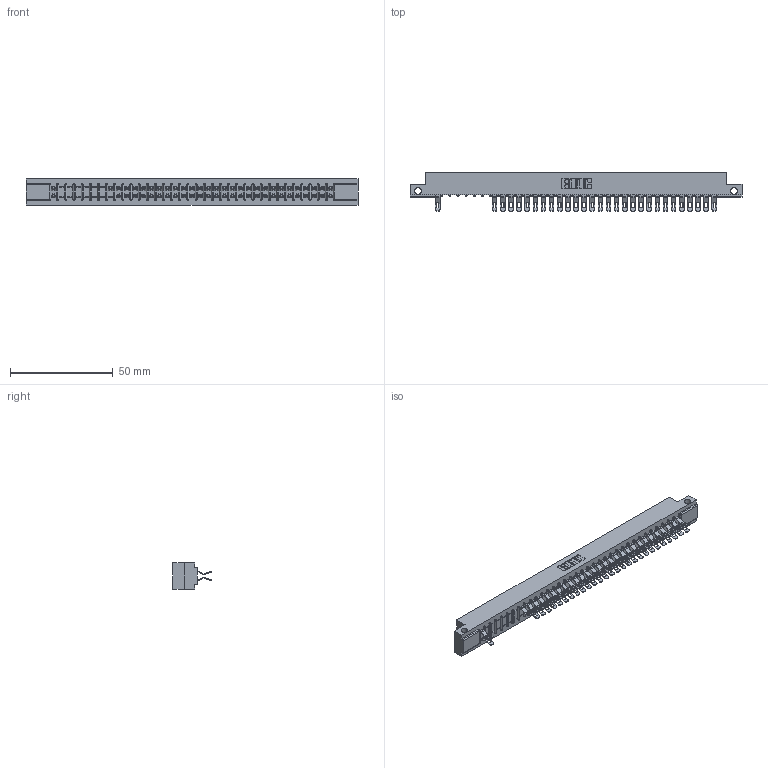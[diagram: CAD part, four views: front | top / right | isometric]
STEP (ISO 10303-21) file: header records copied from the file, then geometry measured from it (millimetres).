
FILE_DESCRIPTION (( 'STEP AP203' ), '1' );
FILE_NAME ('307-070-555-212.STEP', '2018-08-06T13:10:49', ( '' ), ( '' ), 'SwSTEP 2.0', 'SolidWorks 2016', '' );
FILE_SCHEMA (( 'CONFIG_CONTROL_DESIGN' ));
Length unit declared in the file: inch
Products named in the file (3): 307 Part_.128 Dia Side Mounting Holes; 307-290-001_555; 307-070-555-212
Assembly tree (58 placements, depth 2):
  307-070-555-212
    307 Part_.128 Dia Side Mounting Holes
    307-290-001_555  x57
Bounding box: 161.7 x 18.75 x 12.7 mm (x, y, z)
Volume: 17004.3 mm3; surface area: 20487.2 mm2
Topology: 58 solids, 58 shells, 3761 faces, 11056 edges, 7196 vertices
Faces by surface type: plane 2086, cylinder 1603, sphere 72
Entity records: 32111 total; most frequent: CARTESIAN_POINT 5314, ORIENTED_EDGE 5280, DIRECTION 5202, EDGE_CURVE 2640, VECTOR 2010, LINE 2010, VERTEX_POINT 1708, AXIS2_PLACEMENT_3D 1596
